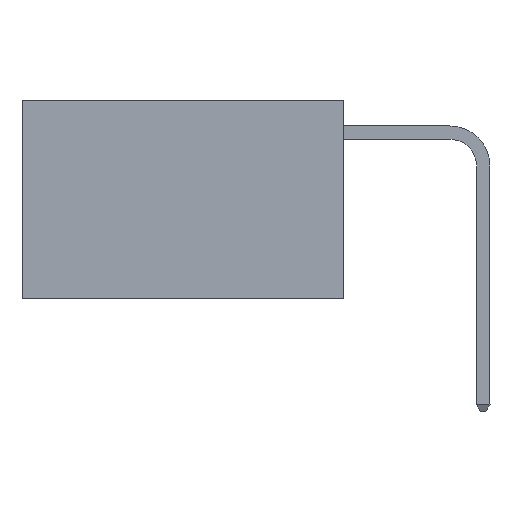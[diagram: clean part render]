
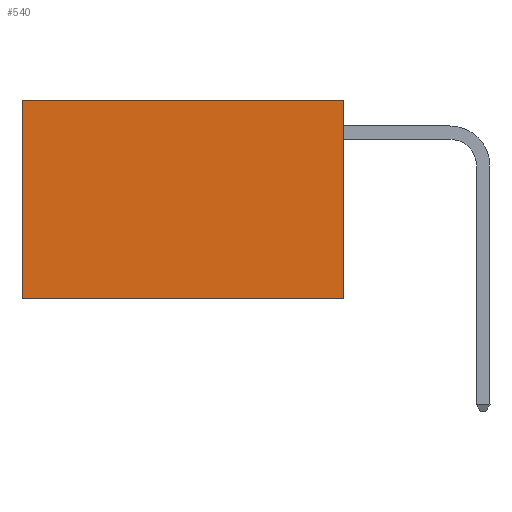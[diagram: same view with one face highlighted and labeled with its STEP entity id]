
A CAD part, left-side view. The second image highlights one B-rep face of the part: STEP entity #540.
In plain terms, the highlighted planar face has unit normal (-1, 0, 0).
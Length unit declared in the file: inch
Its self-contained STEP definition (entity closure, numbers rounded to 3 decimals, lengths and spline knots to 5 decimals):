
#33 = CARTESIAN_POINT ( 'NONE',  ( 0.2625, 0., 0. ) ) ;
#144 = CARTESIAN_POINT ( 'NONE',  ( 0.2625, 0., -0.37 ) ) ;
#158 = VERTEX_POINT ( 'NONE', #8291 ) ;
#540 = ADVANCED_FACE ( 'NONE', ( #3559 ), #9966, .F. ) ;
#874 = DIRECTION ( 'NONE',  ( 0., 0., -1. ) ) ;
#1356 = EDGE_CURVE ( 'NONE', #7828, #158, #5708, .T. ) ;
#1630 = CARTESIAN_POINT ( 'NONE',  ( 0.2625, 0., -0.37 ) ) ;
#2051 = ORIENTED_EDGE ( 'NONE', *, *, #2697, .F. ) ;
#2583 = ORIENTED_EDGE ( 'NONE', *, *, #5322, .T. ) ;
#2637 = LINE ( 'NONE', #5859, #9031 ) ;
#2697 = EDGE_CURVE ( 'NONE', #3548, #7828, #7314, .T. ) ;
#2816 = DIRECTION ( 'NONE',  ( 1., 0., 0. ) ) ;
#3071 = ORIENTED_EDGE ( 'NONE', *, *, #4452, .T. ) ;
#3329 = CARTESIAN_POINT ( 'NONE',  ( 0.2625, 0., 0. ) ) ;
#3548 = VERTEX_POINT ( 'NONE', #6778 ) ;
#3559 = FACE_OUTER_BOUND ( 'NONE', #6740, .T. ) ;
#3659 = DIRECTION ( 'NONE',  ( 0., 0., -1. ) ) ;
#4452 = EDGE_CURVE ( 'NONE', #3548, #5304, #4901, .T. ) ;
#4811 = DIRECTION ( 'NONE',  ( 0., 1., 0. ) ) ;
#4857 = VECTOR ( 'NONE', #4811, 39.37008 ) ;
#4901 = LINE ( 'NONE', #33, #4857 ) ;
#4916 = CARTESIAN_POINT ( 'NONE',  ( 0.2625, 0.6, 0. ) ) ;
#5234 = ORIENTED_EDGE ( 'NONE', *, *, #1356, .F. ) ;
#5304 = VERTEX_POINT ( 'NONE', #4916 ) ;
#5322 = EDGE_CURVE ( 'NONE', #5304, #158, #2637, .T. ) ;
#5506 = AXIS2_PLACEMENT_3D ( 'NONE', #6978, #2816, #3659 ) ;
#5708 = LINE ( 'NONE', #144, #5869 ) ;
#5761 = DIRECTION ( 'NONE',  ( 0., 1., 0. ) ) ;
#5763 = DIRECTION ( 'NONE',  ( 0., 0., -1. ) ) ;
#5859 = CARTESIAN_POINT ( 'NONE',  ( 0.2625, 0.6, 0. ) ) ;
#5869 = VECTOR ( 'NONE', #5761, 39.37008 ) ;
#6414 = VECTOR ( 'NONE', #5763, 39.37008 ) ;
#6740 = EDGE_LOOP ( 'NONE', ( #2583, #5234, #2051, #3071 ) ) ;
#6778 = CARTESIAN_POINT ( 'NONE',  ( 0.2625, 0., 0. ) ) ;
#6978 = CARTESIAN_POINT ( 'NONE',  ( 0.2625, 0., 0. ) ) ;
#7314 = LINE ( 'NONE', #3329, #6414 ) ;
#7828 = VERTEX_POINT ( 'NONE', #1630 ) ;
#8291 = CARTESIAN_POINT ( 'NONE',  ( 0.2625, 0.6, -0.37 ) ) ;
#9031 = VECTOR ( 'NONE', #874, 39.37008 ) ;
#9966 = PLANE ( 'NONE',  #5506 ) ;
